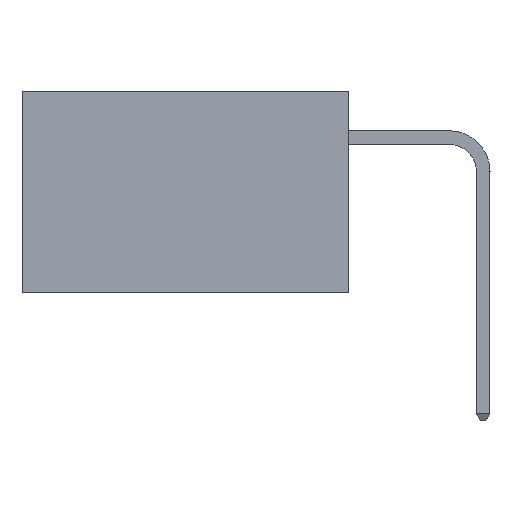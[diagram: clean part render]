
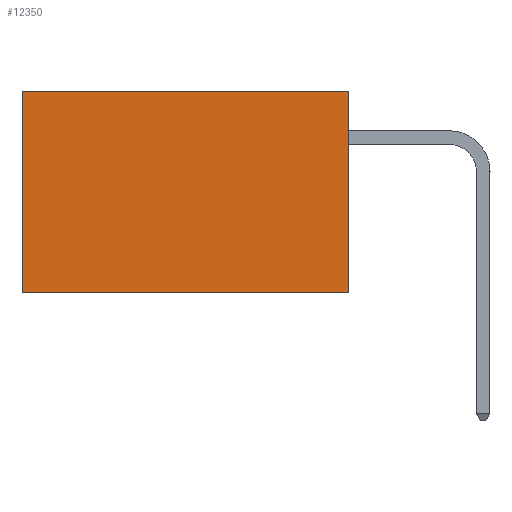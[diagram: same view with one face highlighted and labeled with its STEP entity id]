
A CAD part, left-side view. The second image highlights one B-rep face of the part: STEP entity #12350.
In plain terms, the highlighted planar face has unit normal (-1, 0, 0).
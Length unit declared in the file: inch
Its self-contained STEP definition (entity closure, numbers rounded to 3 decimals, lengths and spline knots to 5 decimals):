
#282 = ORIENTED_EDGE ( 'NONE', *, *, #21887, .F. ) ;
#2987 = DIRECTION ( 'NONE',  ( 0., 0., -1. ) ) ;
#4284 = ORIENTED_EDGE ( 'NONE', *, *, #7384, .F. ) ;
#5760 = VERTEX_POINT ( 'NONE', #27619 ) ;
#7211 = LINE ( 'NONE', #15733, #32336 ) ;
#7384 = EDGE_CURVE ( 'NONE', #17300, #22719, #24156, .T. ) ;
#7994 = CARTESIAN_POINT ( 'NONE',  ( 0.2875, 0., 0. ) ) ;
#9620 = DIRECTION ( 'NONE',  ( 1., 0., 0. ) ) ;
#10801 = VECTOR ( 'NONE', #13548, 39.37008 ) ;
#11348 = EDGE_CURVE ( 'NONE', #5760, #22719, #7211, .T. ) ;
#12350 = ADVANCED_FACE ( 'NONE', ( #15872 ), #17101, .F. ) ;
#12496 = DIRECTION ( 'NONE',  ( 0., 0., -1. ) ) ;
#12645 = VECTOR ( 'NONE', #15656, 39.37008 ) ;
#12986 = LINE ( 'NONE', #7994, #12645 ) ;
#13548 = DIRECTION ( 'NONE',  ( 0., 1., 0. ) ) ;
#15656 = DIRECTION ( 'NONE',  ( 0., 1., 0. ) ) ;
#15733 = CARTESIAN_POINT ( 'NONE',  ( 0.2875, 0.6, 0. ) ) ;
#15872 = FACE_OUTER_BOUND ( 'NONE', #18586, .T. ) ;
#17027 = VECTOR ( 'NONE', #12496, 39.37008 ) ;
#17101 = PLANE ( 'NONE',  #29045 ) ;
#17300 = VERTEX_POINT ( 'NONE', #22229 ) ;
#18438 = CARTESIAN_POINT ( 'NONE',  ( 0.2875, 0., -0.37 ) ) ;
#18586 = EDGE_LOOP ( 'NONE', ( #26698, #4284, #282, #27670 ) ) ;
#19370 = CARTESIAN_POINT ( 'NONE',  ( 0.2875, 0.6, -0.37 ) ) ;
#21887 = EDGE_CURVE ( 'NONE', #27170, #17300, #30286, .T. ) ;
#22229 = CARTESIAN_POINT ( 'NONE',  ( 0.2875, 0., -0.37 ) ) ;
#22351 = CARTESIAN_POINT ( 'NONE',  ( 0.2875, 0., 0. ) ) ;
#22719 = VERTEX_POINT ( 'NONE', #19370 ) ;
#24156 = LINE ( 'NONE', #18438, #10801 ) ;
#25342 = CARTESIAN_POINT ( 'NONE',  ( 0.2875, 0., 0. ) ) ;
#26628 = EDGE_CURVE ( 'NONE', #27170, #5760, #12986, .T. ) ;
#26698 = ORIENTED_EDGE ( 'NONE', *, *, #11348, .T. ) ;
#27166 = DIRECTION ( 'NONE',  ( 0., 0., -1. ) ) ;
#27170 = VERTEX_POINT ( 'NONE', #25342 ) ;
#27619 = CARTESIAN_POINT ( 'NONE',  ( 0.2875, 0.6, 0. ) ) ;
#27670 = ORIENTED_EDGE ( 'NONE', *, *, #26628, .T. ) ;
#29045 = AXIS2_PLACEMENT_3D ( 'NONE', #29537, #9620, #27166 ) ;
#29537 = CARTESIAN_POINT ( 'NONE',  ( 0.2875, 0., 0. ) ) ;
#30286 = LINE ( 'NONE', #22351, #17027 ) ;
#32336 = VECTOR ( 'NONE', #2987, 39.37008 ) ;
